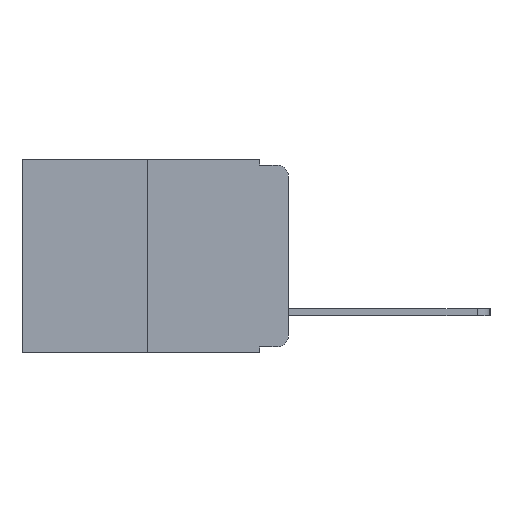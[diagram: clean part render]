
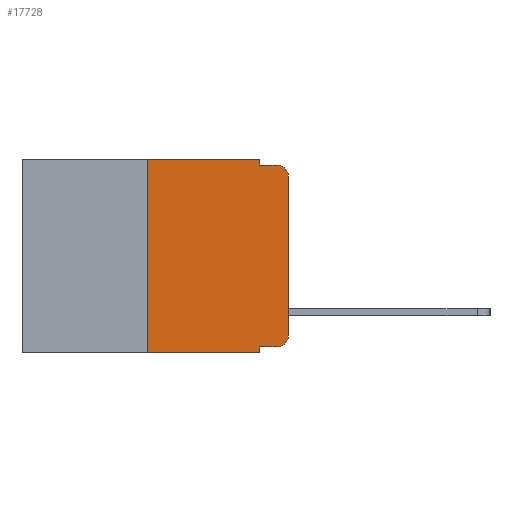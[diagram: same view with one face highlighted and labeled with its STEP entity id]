
A CAD part, left-side view. The second image highlights one B-rep face of the part: STEP entity #17728.
In plain terms, the highlighted planar face has unit normal (-1, 0, 0).
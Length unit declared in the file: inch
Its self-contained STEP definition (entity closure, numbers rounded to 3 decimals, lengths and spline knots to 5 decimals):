
#385 = DIRECTION ( 'NONE',  ( 0., -1., 0. ) ) ;
#728 = EDGE_CURVE ( 'NONE', #3938, #7110, #13898, .T. ) ;
#822 = CARTESIAN_POINT ( 'NONE',  ( 0., 0.051, 0. ) ) ;
#849 = EDGE_CURVE ( 'NONE', #21364, #11343, #20460, .T. ) ;
#893 = AXIS2_PLACEMENT_3D ( 'NONE', #9481, #21592, #11413 ) ;
#930 = VERTEX_POINT ( 'NONE', #21717 ) ;
#1369 = EDGE_CURVE ( 'NONE', #1580, #14489, #20269, .T. ) ;
#1572 = VECTOR ( 'NONE', #6733, 39.37008 ) ;
#1580 = VERTEX_POINT ( 'NONE', #17379 ) ;
#1749 = CARTESIAN_POINT ( 'NONE',  ( 0., 0.051, -0.343 ) ) ;
#1782 = VERTEX_POINT ( 'NONE', #10948 ) ;
#2245 = LINE ( 'NONE', #13632, #10853 ) ;
#2558 = LINE ( 'NONE', #20780, #11779 ) ;
#2683 = CARTESIAN_POINT ( 'NONE',  ( 0., 0., -0.03 ) ) ;
#2990 = EDGE_CURVE ( 'NONE', #7110, #1782, #9563, .T. ) ;
#3412 = VECTOR ( 'NONE', #3605, 39.37008 ) ;
#3436 = EDGE_CURVE ( 'NONE', #14843, #14233, #11338, .T. ) ;
#3605 = DIRECTION ( 'NONE',  ( 0., -1., 0. ) ) ;
#3610 = CARTESIAN_POINT ( 'NONE',  ( 0., 0., 0. ) ) ;
#3749 = DIRECTION ( 'NONE',  ( 0., 0., 1. ) ) ;
#3796 = AXIS2_PLACEMENT_3D ( 'NONE', #16166, #5484, #17876 ) ;
#3938 = VERTEX_POINT ( 'NONE', #5479 ) ;
#4231 = ORIENTED_EDGE ( 'NONE', *, *, #728, .T. ) ;
#4257 = ORIENTED_EDGE ( 'NONE', *, *, #3436, .F. ) ;
#4950 = ORIENTED_EDGE ( 'NONE', *, *, #18359, .T. ) ;
#5479 = CARTESIAN_POINT ( 'NONE',  ( 0., 0., -0.313 ) ) ;
#5484 = DIRECTION ( 'NONE',  ( -1., 0., 0. ) ) ;
#5980 = CARTESIAN_POINT ( 'NONE',  ( 0., 0.25, 0. ) ) ;
#6301 = DIRECTION ( 'NONE',  ( 0., -1., 0. ) ) ;
#6336 = VECTOR ( 'NONE', #22400, 39.37008 ) ;
#6733 = DIRECTION ( 'NONE',  ( 0., 0., 1. ) ) ;
#7110 = VERTEX_POINT ( 'NONE', #2683 ) ;
#8258 = LINE ( 'NONE', #19487, #3412 ) ;
#8376 = VECTOR ( 'NONE', #385, 39.37008 ) ;
#8470 = DIRECTION ( 'NONE',  ( 0., 0., -1. ) ) ;
#8990 = VECTOR ( 'NONE', #3749, 39.37008 ) ;
#9481 = CARTESIAN_POINT ( 'NONE',  ( 0., 0.473, 0. ) ) ;
#9524 = EDGE_CURVE ( 'NONE', #14233, #1782, #2558, .T. ) ;
#9563 = CIRCLE ( 'NONE', #13849, 0.02 ) ;
#9638 = CARTESIAN_POINT ( 'NONE',  ( 0., 0.051, -0.333 ) ) ;
#9641 = CARTESIAN_POINT ( 'NONE',  ( 0., 0.051, 0. ) ) ;
#9689 = EDGE_CURVE ( 'NONE', #11343, #14843, #8258, .T. ) ;
#10739 = EDGE_CURVE ( 'NONE', #21364, #14489, #2245, .T. ) ;
#10853 = VECTOR ( 'NONE', #6301, 39.37008 ) ;
#10948 = CARTESIAN_POINT ( 'NONE',  ( 0., 0.02, -0.01 ) ) ;
#11159 = CARTESIAN_POINT ( 'NONE',  ( 0., 0.051, -0.01 ) ) ;
#11338 = LINE ( 'NONE', #9641, #15980 ) ;
#11343 = VERTEX_POINT ( 'NONE', #11991 ) ;
#11381 = ORIENTED_EDGE ( 'NONE', *, *, #2990, .T. ) ;
#11413 = DIRECTION ( 'NONE',  ( 0., 0., -1. ) ) ;
#11779 = VECTOR ( 'NONE', #12308, 39.37008 ) ;
#11991 = CARTESIAN_POINT ( 'NONE',  ( 0., 0.25, 0. ) ) ;
#12308 = DIRECTION ( 'NONE',  ( 0., -1., 0. ) ) ;
#12470 = CIRCLE ( 'NONE', #3796, 0.02 ) ;
#12583 = EDGE_LOOP ( 'NONE', ( #4231, #11381, #15784, #4257, #19444, #22008, #20265, #12899, #16098, #4950 ) ) ;
#12899 = ORIENTED_EDGE ( 'NONE', *, *, #1369, .F. ) ;
#13314 = LINE ( 'NONE', #9638, #8376 ) ;
#13632 = CARTESIAN_POINT ( 'NONE',  ( 0., 0.473, -0.343 ) ) ;
#13849 = AXIS2_PLACEMENT_3D ( 'NONE', #14636, #14629, #15837 ) ;
#13898 = LINE ( 'NONE', #3610, #8990 ) ;
#14233 = VERTEX_POINT ( 'NONE', #11159 ) ;
#14489 = VERTEX_POINT ( 'NONE', #1749 ) ;
#14629 = DIRECTION ( 'NONE',  ( -1., 0., 0. ) ) ;
#14636 = CARTESIAN_POINT ( 'NONE',  ( 0., 0.02, -0.03 ) ) ;
#14843 = VERTEX_POINT ( 'NONE', #20355 ) ;
#15784 = ORIENTED_EDGE ( 'NONE', *, *, #9524, .F. ) ;
#15837 = DIRECTION ( 'NONE',  ( 0., 0., -1. ) ) ;
#15980 = VECTOR ( 'NONE', #8470, 39.37008 ) ;
#16098 = ORIENTED_EDGE ( 'NONE', *, *, #18649, .T. ) ;
#16166 = CARTESIAN_POINT ( 'NONE',  ( 0., 0.02, -0.313 ) ) ;
#16504 = FACE_OUTER_BOUND ( 'NONE', #12583, .T. ) ;
#17379 = CARTESIAN_POINT ( 'NONE',  ( 0., 0.051, -0.333 ) ) ;
#17728 = ADVANCED_FACE ( 'NONE', ( #16504 ), #18256, .F. ) ;
#17876 = DIRECTION ( 'NONE',  ( 0., 0., -1. ) ) ;
#18256 = PLANE ( 'NONE',  #893 ) ;
#18359 = EDGE_CURVE ( 'NONE', #930, #3938, #12470, .T. ) ;
#18649 = EDGE_CURVE ( 'NONE', #1580, #930, #13314, .T. ) ;
#19444 = ORIENTED_EDGE ( 'NONE', *, *, #9689, .F. ) ;
#19487 = CARTESIAN_POINT ( 'NONE',  ( 0., 0.473, 0. ) ) ;
#19985 = CARTESIAN_POINT ( 'NONE',  ( 0., 0.25, -0.343 ) ) ;
#20265 = ORIENTED_EDGE ( 'NONE', *, *, #10739, .T. ) ;
#20269 = LINE ( 'NONE', #822, #6336 ) ;
#20355 = CARTESIAN_POINT ( 'NONE',  ( 0., 0.051, 0. ) ) ;
#20460 = LINE ( 'NONE', #5980, #1572 ) ;
#20780 = CARTESIAN_POINT ( 'NONE',  ( 0., 0.051, -0.01 ) ) ;
#21364 = VERTEX_POINT ( 'NONE', #19985 ) ;
#21592 = DIRECTION ( 'NONE',  ( 1., 0., 0. ) ) ;
#21717 = CARTESIAN_POINT ( 'NONE',  ( 0., 0.02, -0.333 ) ) ;
#22008 = ORIENTED_EDGE ( 'NONE', *, *, #849, .F. ) ;
#22400 = DIRECTION ( 'NONE',  ( 0., 0., -1. ) ) ;
